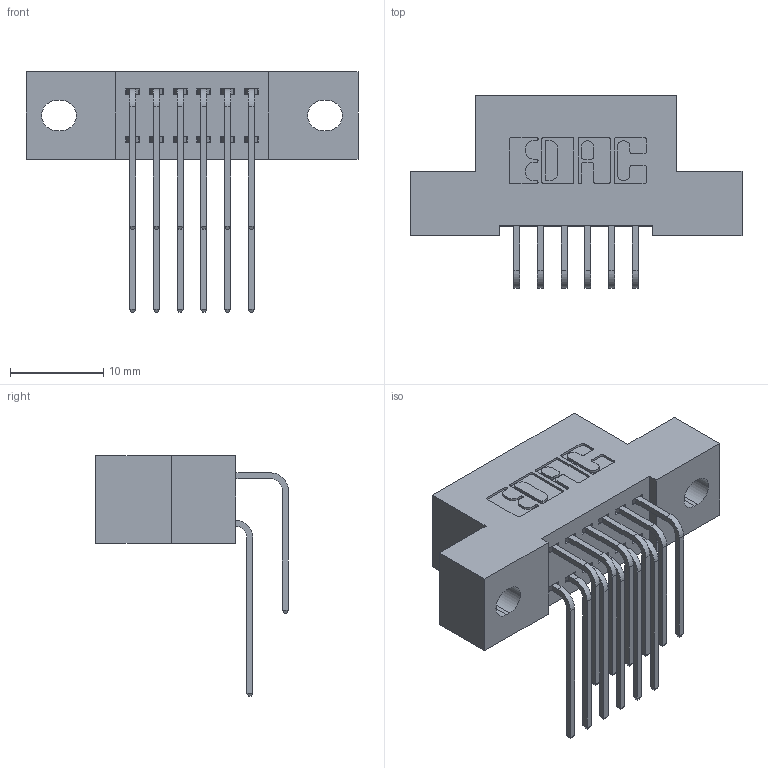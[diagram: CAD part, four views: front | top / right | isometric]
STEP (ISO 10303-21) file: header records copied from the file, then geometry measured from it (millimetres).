
FILE_DESCRIPTION (( 'STEP AP203' ), '1' );
FILE_NAME ('392-012-559-202.STEP', '2019-10-07T01:43:53', ( '' ), ( '' ), 'SwSTEP 2.0', 'SolidWorks 2016', '' );
FILE_SCHEMA (( 'CONFIG_CONTROL_DESIGN' ));
Length unit declared in the file: inch
Products named in the file (4): 342 Part_.128 Slot; 345-292-001_558 559 Tail - 1; 345-292-001_559 Tail - 2; 392-012-559-202
Assembly tree (13 placements, depth 2):
  392-012-559-202
    342 Part_.128 Slot
    345-292-001_558 559 Tail - 1  x6
    345-292-001_559 Tail - 2  x6
Bounding box: 35.56 x 20.64 x 25.78 mm (x, y, z)
Volume: 3041.7 mm3; surface area: 4136.8 mm2
Topology: 13 solids, 13 shells, 762 faces, 2243 edges, 1478 vertices
Faces by surface type: plane 526, cylinder 236
Entity records: 10303 total; most frequent: CARTESIAN_POINT 1801, ORIENTED_EDGE 1686, DIRECTION 1583, EDGE_CURVE 843, LINE 675, VECTOR 675, VERTEX_POINT 558, AXIS2_PLACEMENT_3D 454
